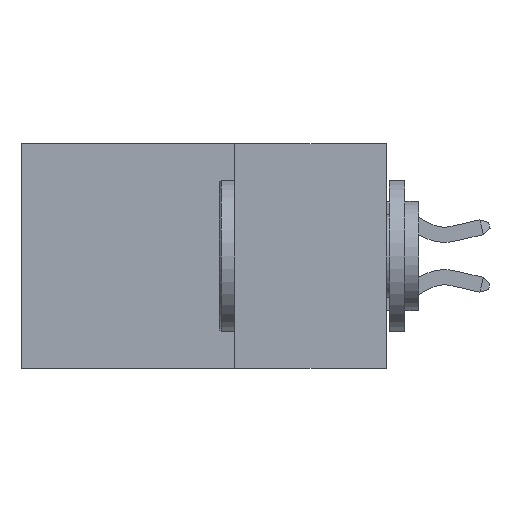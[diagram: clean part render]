
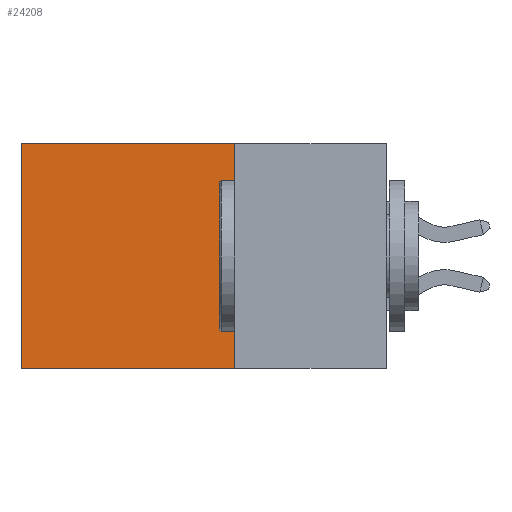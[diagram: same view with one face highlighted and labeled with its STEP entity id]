
A CAD part, left-side view. The second image highlights one B-rep face of the part: STEP entity #24208.
In plain terms, the highlighted planar face has unit normal (-1, 0, 0).
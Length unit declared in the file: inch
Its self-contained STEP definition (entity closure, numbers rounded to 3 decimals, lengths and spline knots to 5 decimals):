
#2266 = CARTESIAN_POINT ( 'NONE',  ( 0.2615, 0.6, -0.37 ) ) ;
#2454 = ORIENTED_EDGE ( 'NONE', *, *, #5291, .F. ) ;
#2832 = DIRECTION ( 'NONE',  ( 0., 0., -1. ) ) ;
#3047 = CARTESIAN_POINT ( 'NONE',  ( 0.2615, 0.25, 0. ) ) ;
#4061 = EDGE_LOOP ( 'NONE', ( #20707, #2454, #15500, #7793 ) ) ;
#4391 = EDGE_CURVE ( 'NONE', #8746, #23846, #17466, .T. ) ;
#5152 = AXIS2_PLACEMENT_3D ( 'NONE', #9366, #21405, #15793 ) ;
#5291 = EDGE_CURVE ( 'NONE', #23601, #19600, #7625, .T. ) ;
#5485 = CARTESIAN_POINT ( 'NONE',  ( 0.2615, 0.6, -0.37 ) ) ;
#5600 = CARTESIAN_POINT ( 'NONE',  ( 0.2615, 0.6, 0. ) ) ;
#5911 = CARTESIAN_POINT ( 'NONE',  ( 0.2615, 0.25, -0.37 ) ) ;
#6899 = LINE ( 'NONE', #11336, #17474 ) ;
#7216 = VECTOR ( 'NONE', #7763, 39.37008 ) ;
#7463 = DIRECTION ( 'NONE',  ( 0., 0., -1. ) ) ;
#7625 = LINE ( 'NONE', #5911, #7216 ) ;
#7763 = DIRECTION ( 'NONE',  ( 0., 1., 0. ) ) ;
#7793 = ORIENTED_EDGE ( 'NONE', *, *, #4391, .T. ) ;
#7919 = FACE_OUTER_BOUND ( 'NONE', #4061, .T. ) ;
#8746 = VERTEX_POINT ( 'NONE', #16615 ) ;
#9366 = CARTESIAN_POINT ( 'NONE',  ( 0.2615, 0.25, -0.37 ) ) ;
#11336 = CARTESIAN_POINT ( 'NONE',  ( 0.2615, 0.25, -0.37 ) ) ;
#13480 = LINE ( 'NONE', #5485, #14448 ) ;
#13947 = PLANE ( 'NONE',  #5152 ) ;
#14448 = VECTOR ( 'NONE', #7463, 39.37008 ) ;
#15500 = ORIENTED_EDGE ( 'NONE', *, *, #20645, .F. ) ;
#15793 = DIRECTION ( 'NONE',  ( 0., 0., -1. ) ) ;
#16615 = CARTESIAN_POINT ( 'NONE',  ( 0.2615, 0.25, 0. ) ) ;
#17451 = EDGE_CURVE ( 'NONE', #23846, #19600, #13480, .T. ) ;
#17466 = LINE ( 'NONE', #3047, #22213 ) ;
#17474 = VECTOR ( 'NONE', #2832, 39.37008 ) ;
#19600 = VERTEX_POINT ( 'NONE', #2266 ) ;
#20645 = EDGE_CURVE ( 'NONE', #8746, #23601, #6899, .T. ) ;
#20707 = ORIENTED_EDGE ( 'NONE', *, *, #17451, .T. ) ;
#21254 = DIRECTION ( 'NONE',  ( 0., 1., 0. ) ) ;
#21405 = DIRECTION ( 'NONE',  ( 1., 0., 0. ) ) ;
#22213 = VECTOR ( 'NONE', #21254, 39.37008 ) ;
#23281 = CARTESIAN_POINT ( 'NONE',  ( 0.2615, 0.25, -0.37 ) ) ;
#23601 = VERTEX_POINT ( 'NONE', #23281 ) ;
#23846 = VERTEX_POINT ( 'NONE', #5600 ) ;
#24208 = ADVANCED_FACE ( 'NONE', ( #7919 ), #13947, .F. ) ;
